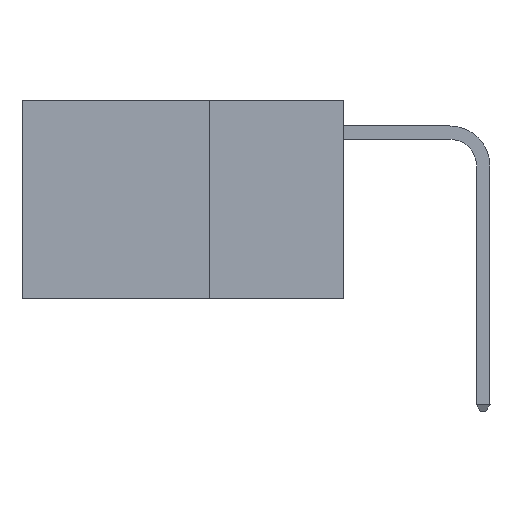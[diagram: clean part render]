
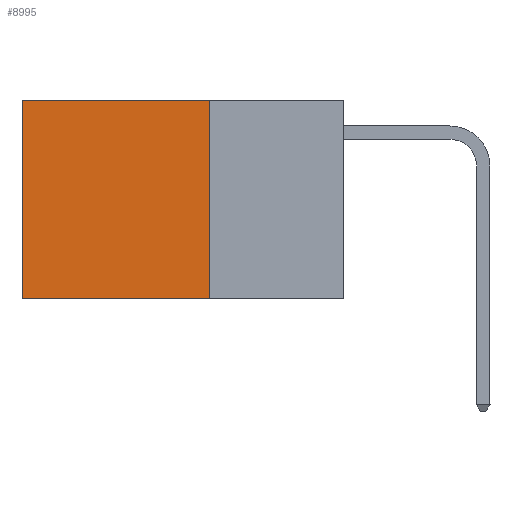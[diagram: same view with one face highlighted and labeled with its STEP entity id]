
A CAD part, left-side view. The second image highlights one B-rep face of the part: STEP entity #8995.
In plain terms, the highlighted planar face has unit normal (-1, 0, 0).
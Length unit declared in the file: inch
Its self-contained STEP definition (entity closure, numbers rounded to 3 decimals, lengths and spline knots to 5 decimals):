
#662 = EDGE_CURVE ( 'NONE', #1087, #1267, #7030, .T. ) ;
#768 = VECTOR ( 'NONE', #3009, 39.37008 ) ;
#886 = AXIS2_PLACEMENT_3D ( 'NONE', #8849, #7124, #7963 ) ;
#1087 = VERTEX_POINT ( 'NONE', #3489 ) ;
#1214 = LINE ( 'NONE', #3605, #768 ) ;
#1267 = VERTEX_POINT ( 'NONE', #9215 ) ;
#1429 = PLANE ( 'NONE',  #886 ) ;
#1867 = EDGE_CURVE ( 'NONE', #1267, #8505, #2659, .T. ) ;
#2040 = ORIENTED_EDGE ( 'NONE', *, *, #8683, .F. ) ;
#2130 = ORIENTED_EDGE ( 'NONE', *, *, #2810, .F. ) ;
#2216 = ORIENTED_EDGE ( 'NONE', *, *, #662, .T. ) ;
#2358 = ORIENTED_EDGE ( 'NONE', *, *, #1867, .T. ) ;
#2645 = VECTOR ( 'NONE', #6271, 39.37008 ) ;
#2659 = LINE ( 'NONE', #6314, #2645 ) ;
#2810 = EDGE_CURVE ( 'NONE', #1087, #7145, #1214, .T. ) ;
#3009 = DIRECTION ( 'NONE',  ( 0., 0., -1. ) ) ;
#3184 = LINE ( 'NONE', #6805, #3195 ) ;
#3195 = VECTOR ( 'NONE', #9025, 39.37008 ) ;
#3489 = CARTESIAN_POINT ( 'NONE',  ( 0.2625, 0.25, 0. ) ) ;
#3605 = CARTESIAN_POINT ( 'NONE',  ( 0.2625, 0.25, 0. ) ) ;
#3835 = CARTESIAN_POINT ( 'NONE',  ( 0.2625, 0.6, -0.37 ) ) ;
#4724 = CARTESIAN_POINT ( 'NONE',  ( 0.2625, 0.25, 0. ) ) ;
#4922 = EDGE_LOOP ( 'NONE', ( #2358, #2040, #2130, #2216 ) ) ;
#6271 = DIRECTION ( 'NONE',  ( 0., 0., -1. ) ) ;
#6314 = CARTESIAN_POINT ( 'NONE',  ( 0.2625, 0.6, 0. ) ) ;
#6658 = CARTESIAN_POINT ( 'NONE',  ( 0.2625, 0.25, -0.37 ) ) ;
#6805 = CARTESIAN_POINT ( 'NONE',  ( 0.2625, 0.25, -0.37 ) ) ;
#6994 = VECTOR ( 'NONE', #8265, 39.37008 ) ;
#7030 = LINE ( 'NONE', #4724, #6994 ) ;
#7124 = DIRECTION ( 'NONE',  ( 1., 0., 0. ) ) ;
#7145 = VERTEX_POINT ( 'NONE', #6658 ) ;
#7963 = DIRECTION ( 'NONE',  ( 0., 0., -1. ) ) ;
#8265 = DIRECTION ( 'NONE',  ( 0., 1., 0. ) ) ;
#8505 = VERTEX_POINT ( 'NONE', #3835 ) ;
#8683 = EDGE_CURVE ( 'NONE', #7145, #8505, #3184, .T. ) ;
#8849 = CARTESIAN_POINT ( 'NONE',  ( 0.2625, 0.25, 0. ) ) ;
#8856 = FACE_OUTER_BOUND ( 'NONE', #4922, .T. ) ;
#8995 = ADVANCED_FACE ( 'NONE', ( #8856 ), #1429, .F. ) ;
#9025 = DIRECTION ( 'NONE',  ( 0., 1., 0. ) ) ;
#9215 = CARTESIAN_POINT ( 'NONE',  ( 0.2625, 0.6, 0. ) ) ;
